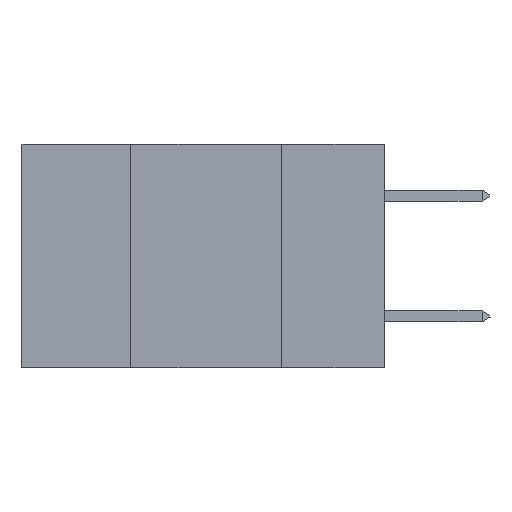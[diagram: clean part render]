
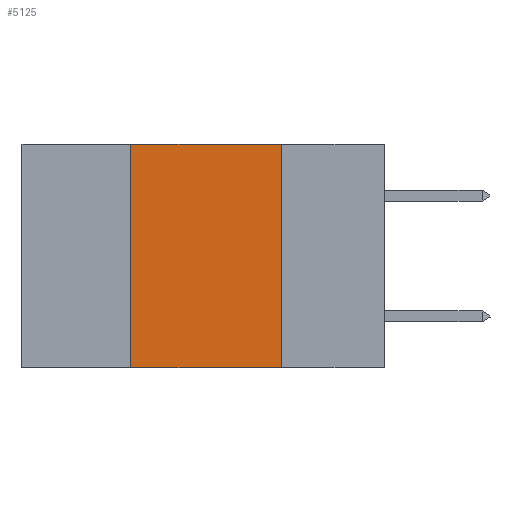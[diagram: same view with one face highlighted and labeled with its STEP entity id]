
A CAD part, left-side view. The second image highlights one B-rep face of the part: STEP entity #5125.
In plain terms, the highlighted planar face has unit normal (-1, 0, 0).
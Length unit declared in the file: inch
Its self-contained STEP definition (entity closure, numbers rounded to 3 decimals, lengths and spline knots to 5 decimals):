
#333 = VECTOR ( 'NONE', #15251, 39.37008 ) ;
#579 = DIRECTION ( 'NONE',  ( 0., 0., -1. ) ) ;
#984 = DIRECTION ( 'NONE',  ( 0., 0., -1. ) ) ;
#2064 = EDGE_LOOP ( 'NONE', ( #18574, #5060, #7426, #9952 ) ) ;
#2978 = VERTEX_POINT ( 'NONE', #13676 ) ;
#3388 = CARTESIAN_POINT ( 'NONE',  ( 0., 0.17, -0.37 ) ) ;
#4059 = VERTEX_POINT ( 'NONE', #23172 ) ;
#4317 = CARTESIAN_POINT ( 'NONE',  ( 0., 0.17, 0. ) ) ;
#5060 = ORIENTED_EDGE ( 'NONE', *, *, #17302, .F. ) ;
#5125 = ADVANCED_FACE ( 'NONE', ( #8465 ), #21115, .F. ) ;
#5231 = LINE ( 'NONE', #7922, #9188 ) ;
#5785 = VECTOR ( 'NONE', #984, 39.37008 ) ;
#5838 = CARTESIAN_POINT ( 'NONE',  ( 0., 0.42, 0. ) ) ;
#6703 = VECTOR ( 'NONE', #13616, 39.37008 ) ;
#6822 = VERTEX_POINT ( 'NONE', #3388 ) ;
#7124 = EDGE_CURVE ( 'NONE', #12311, #2978, #16204, .T. ) ;
#7426 = ORIENTED_EDGE ( 'NONE', *, *, #7124, .F. ) ;
#7833 = DIRECTION ( 'NONE',  ( 0., -1., 0. ) ) ;
#7922 = CARTESIAN_POINT ( 'NONE',  ( 0., 0.6, 0. ) ) ;
#8465 = FACE_OUTER_BOUND ( 'NONE', #2064, .T. ) ;
#9188 = VECTOR ( 'NONE', #7833, 39.37008 ) ;
#9625 = CARTESIAN_POINT ( 'NONE',  ( 0., 0.6, 0. ) ) ;
#9952 = ORIENTED_EDGE ( 'NONE', *, *, #19167, .T. ) ;
#12311 = VERTEX_POINT ( 'NONE', #23470 ) ;
#13616 = DIRECTION ( 'NONE',  ( 0., -1., 0. ) ) ;
#13676 = CARTESIAN_POINT ( 'NONE',  ( 0., 0.42, 0. ) ) ;
#15251 = DIRECTION ( 'NONE',  ( 0., 0., 1. ) ) ;
#16204 = LINE ( 'NONE', #5838, #333 ) ;
#16358 = AXIS2_PLACEMENT_3D ( 'NONE', #9625, #23041, #579 ) ;
#16948 = LINE ( 'NONE', #18863, #6703 ) ;
#17302 = EDGE_CURVE ( 'NONE', #2978, #4059, #5231, .T. ) ;
#18574 = ORIENTED_EDGE ( 'NONE', *, *, #19441, .F. ) ;
#18863 = CARTESIAN_POINT ( 'NONE',  ( 0., 0.6, -0.37 ) ) ;
#19167 = EDGE_CURVE ( 'NONE', #12311, #6822, #16948, .T. ) ;
#19441 = EDGE_CURVE ( 'NONE', #4059, #6822, #21113, .T. ) ;
#21113 = LINE ( 'NONE', #4317, #5785 ) ;
#21115 = PLANE ( 'NONE',  #16358 ) ;
#23041 = DIRECTION ( 'NONE',  ( 1., 0., 0. ) ) ;
#23172 = CARTESIAN_POINT ( 'NONE',  ( 0., 0.17, 0. ) ) ;
#23470 = CARTESIAN_POINT ( 'NONE',  ( 0., 0.42, -0.37 ) ) ;
